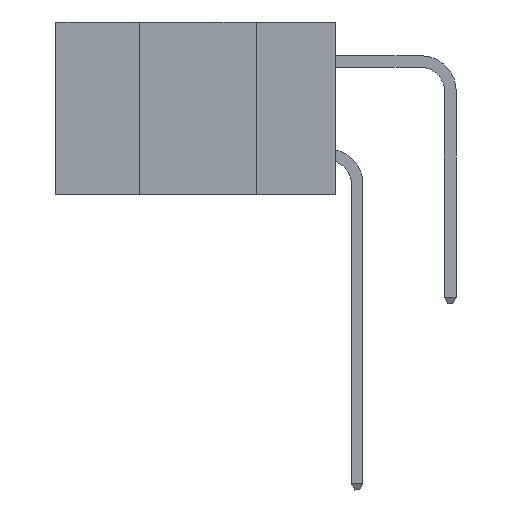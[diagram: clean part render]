
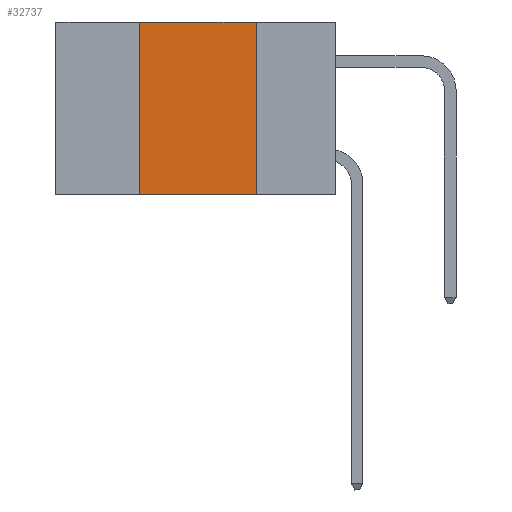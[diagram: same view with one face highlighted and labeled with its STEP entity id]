
A CAD part, left-side view. The second image highlights one B-rep face of the part: STEP entity #32737.
In plain terms, the highlighted planar face has unit normal (-1, 0, 0).
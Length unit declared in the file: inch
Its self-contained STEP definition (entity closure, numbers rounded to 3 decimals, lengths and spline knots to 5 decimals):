
#911 = EDGE_CURVE ( 'NONE', #2263, #4262, #11978, .T. ) ;
#1887 = ORIENTED_EDGE ( 'NONE', *, *, #911, .F. ) ;
#1953 = VERTEX_POINT ( 'NONE', #32186 ) ;
#2263 = VERTEX_POINT ( 'NONE', #17538 ) ;
#3505 = LINE ( 'NONE', #11814, #33776 ) ;
#3857 = FACE_OUTER_BOUND ( 'NONE', #23930, .T. ) ;
#4262 = VERTEX_POINT ( 'NONE', #27576 ) ;
#4784 = CARTESIAN_POINT ( 'NONE',  ( 0., 0.6, -0.37 ) ) ;
#6680 = EDGE_CURVE ( 'NONE', #17796, #1953, #22681, .T. ) ;
#6805 = CARTESIAN_POINT ( 'NONE',  ( 0., 0.42, 0. ) ) ;
#6932 = ORIENTED_EDGE ( 'NONE', *, *, #20038, .T. ) ;
#10545 = VECTOR ( 'NONE', #29329, 39.37008 ) ;
#11814 = CARTESIAN_POINT ( 'NONE',  ( 0., 0.6, 0. ) ) ;
#11978 = LINE ( 'NONE', #6805, #10545 ) ;
#13040 = AXIS2_PLACEMENT_3D ( 'NONE', #26391, #20845, #35053 ) ;
#15117 = PLANE ( 'NONE',  #13040 ) ;
#15499 = DIRECTION ( 'NONE',  ( 0., -1., 0. ) ) ;
#16663 = ORIENTED_EDGE ( 'NONE', *, *, #6680, .F. ) ;
#16957 = DIRECTION ( 'NONE',  ( 0., 0., -1. ) ) ;
#17538 = CARTESIAN_POINT ( 'NONE',  ( 0., 0.42, -0.37 ) ) ;
#17796 = VERTEX_POINT ( 'NONE', #29896 ) ;
#19728 = CARTESIAN_POINT ( 'NONE',  ( 0., 0.17, 0. ) ) ;
#20038 = EDGE_CURVE ( 'NONE', #2263, #1953, #26964, .T. ) ;
#20845 = DIRECTION ( 'NONE',  ( 1., 0., 0. ) ) ;
#22681 = LINE ( 'NONE', #19728, #32769 ) ;
#23086 = DIRECTION ( 'NONE',  ( 0., -1., 0. ) ) ;
#23930 = EDGE_LOOP ( 'NONE', ( #16663, #35365, #1887, #6932 ) ) ;
#26391 = CARTESIAN_POINT ( 'NONE',  ( 0., 0.6, 0. ) ) ;
#26964 = LINE ( 'NONE', #4784, #32767 ) ;
#27576 = CARTESIAN_POINT ( 'NONE',  ( 0., 0.42, 0. ) ) ;
#29329 = DIRECTION ( 'NONE',  ( 0., 0., 1. ) ) ;
#29896 = CARTESIAN_POINT ( 'NONE',  ( 0., 0.17, 0. ) ) ;
#32186 = CARTESIAN_POINT ( 'NONE',  ( 0., 0.17, -0.37 ) ) ;
#32737 = ADVANCED_FACE ( 'NONE', ( #3857 ), #15117, .F. ) ;
#32767 = VECTOR ( 'NONE', #15499, 39.37008 ) ;
#32769 = VECTOR ( 'NONE', #16957, 39.37008 ) ;
#33776 = VECTOR ( 'NONE', #23086, 39.37008 ) ;
#33906 = EDGE_CURVE ( 'NONE', #4262, #17796, #3505, .T. ) ;
#35053 = DIRECTION ( 'NONE',  ( 0., 0., -1. ) ) ;
#35365 = ORIENTED_EDGE ( 'NONE', *, *, #33906, .F. ) ;
